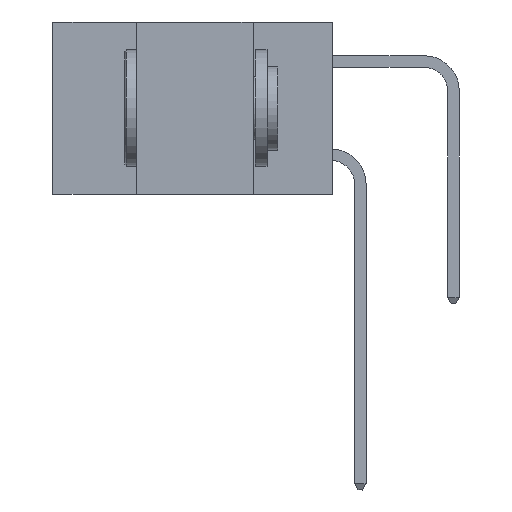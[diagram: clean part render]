
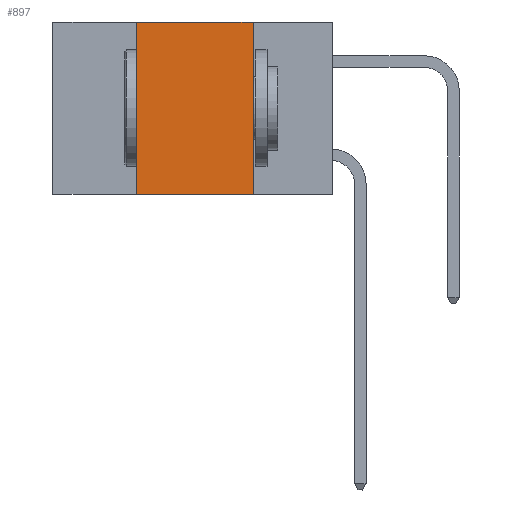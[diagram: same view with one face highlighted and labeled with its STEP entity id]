
A CAD part, left-side view. The second image highlights one B-rep face of the part: STEP entity #897.
In plain terms, the highlighted planar face has unit normal (-1, 0, 0).
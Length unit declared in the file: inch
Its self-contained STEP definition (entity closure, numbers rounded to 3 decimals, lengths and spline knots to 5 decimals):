
#102 = CARTESIAN_POINT ( 'NONE',  ( 0., 0.17, -0.37 ) ) ;
#639 = ORIENTED_EDGE ( 'NONE', *, *, #15905, .F. ) ;
#730 = VECTOR ( 'NONE', #18061, 39.37008 ) ;
#897 = ADVANCED_FACE ( 'NONE', ( #6763 ), #13706, .F. ) ;
#2452 = DIRECTION ( 'NONE',  ( 0., 0., -1. ) ) ;
#3304 = DIRECTION ( 'NONE',  ( 0., -1., 0. ) ) ;
#3532 = ORIENTED_EDGE ( 'NONE', *, *, #12100, .F. ) ;
#3756 = VERTEX_POINT ( 'NONE', #4119 ) ;
#3806 = DIRECTION ( 'NONE',  ( 1., 0., 0. ) ) ;
#4119 = CARTESIAN_POINT ( 'NONE',  ( 0., 0.42, 0. ) ) ;
#4388 = VECTOR ( 'NONE', #16562, 39.37008 ) ;
#4518 = EDGE_CURVE ( 'NONE', #7607, #17856, #11059, .T. ) ;
#5059 = LINE ( 'NONE', #12125, #11063 ) ;
#5204 = DIRECTION ( 'NONE',  ( 0., 0., -1. ) ) ;
#6763 = FACE_OUTER_BOUND ( 'NONE', #10759, .T. ) ;
#7607 = VERTEX_POINT ( 'NONE', #15683 ) ;
#7689 = LINE ( 'NONE', #13119, #4388 ) ;
#8137 = CARTESIAN_POINT ( 'NONE',  ( 0., 0.6, 0. ) ) ;
#8442 = ORIENTED_EDGE ( 'NONE', *, *, #4518, .T. ) ;
#9658 = CARTESIAN_POINT ( 'NONE',  ( 0., 0.6, 0. ) ) ;
#10090 = CARTESIAN_POINT ( 'NONE',  ( 0., 0.17, 0. ) ) ;
#10661 = VERTEX_POINT ( 'NONE', #10090 ) ;
#10759 = EDGE_LOOP ( 'NONE', ( #14320, #3532, #639, #8442 ) ) ;
#11059 = LINE ( 'NONE', #17478, #12357 ) ;
#11063 = VECTOR ( 'NONE', #2452, 39.37008 ) ;
#12100 = EDGE_CURVE ( 'NONE', #3756, #10661, #17362, .T. ) ;
#12125 = CARTESIAN_POINT ( 'NONE',  ( 0., 0.17, 0. ) ) ;
#12357 = VECTOR ( 'NONE', #3304, 39.37008 ) ;
#13119 = CARTESIAN_POINT ( 'NONE',  ( 0., 0.42, 0. ) ) ;
#13706 = PLANE ( 'NONE',  #16174 ) ;
#14320 = ORIENTED_EDGE ( 'NONE', *, *, #14749, .F. ) ;
#14749 = EDGE_CURVE ( 'NONE', #10661, #17856, #5059, .T. ) ;
#15683 = CARTESIAN_POINT ( 'NONE',  ( 0., 0.42, -0.37 ) ) ;
#15905 = EDGE_CURVE ( 'NONE', #7607, #3756, #7689, .T. ) ;
#16174 = AXIS2_PLACEMENT_3D ( 'NONE', #9658, #3806, #5204 ) ;
#16562 = DIRECTION ( 'NONE',  ( 0., 0., 1. ) ) ;
#17362 = LINE ( 'NONE', #8137, #730 ) ;
#17478 = CARTESIAN_POINT ( 'NONE',  ( 0., 0.6, -0.37 ) ) ;
#17856 = VERTEX_POINT ( 'NONE', #102 ) ;
#18061 = DIRECTION ( 'NONE',  ( 0., -1., 0. ) ) ;
